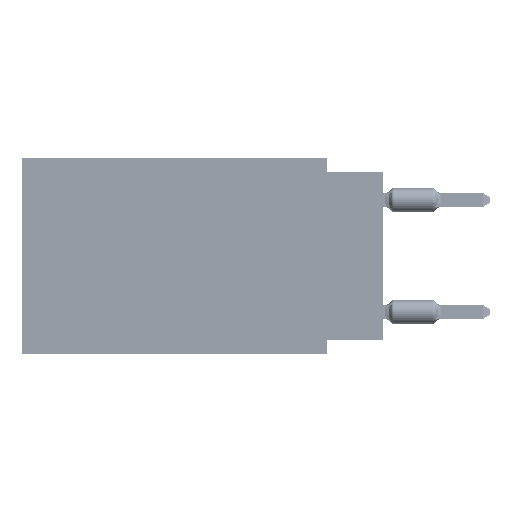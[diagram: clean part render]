
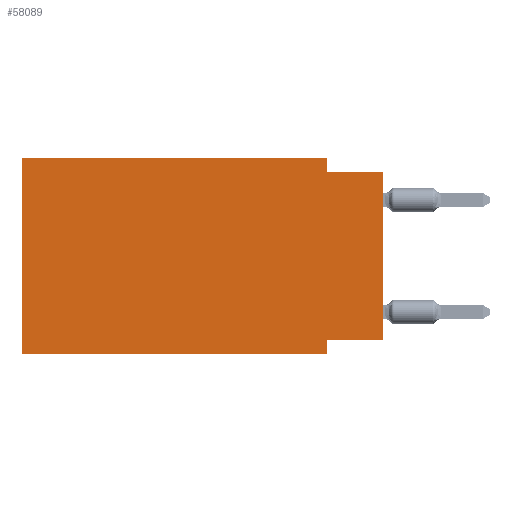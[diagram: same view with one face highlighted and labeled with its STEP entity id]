
A CAD part, left-side view. The second image highlights one B-rep face of the part: STEP entity #58089.
In plain terms, the highlighted planar face has unit normal (-1, 0, 0).
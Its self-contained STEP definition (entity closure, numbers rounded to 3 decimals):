
#378 = PLANE ( 'NONE',  #42816 ) ;
#550 = DIRECTION ( 'NONE',  ( 0., -1., 0. ) ) ;
#5020 = VERTEX_POINT ( 'NONE', #30800 ) ;
#8873 = CARTESIAN_POINT ( 'NONE',  ( 0., 0., -8.255 ) ) ;
#9636 = VECTOR ( 'NONE', #550, 1000. ) ;
#10598 = CARTESIAN_POINT ( 'NONE',  ( 0., 16.383, 0. ) ) ;
#11968 = DIRECTION ( 'NONE',  ( 0., -1., 0. ) ) ;
#13054 = VERTEX_POINT ( 'NONE', #8873 ) ;
#13843 = CARTESIAN_POINT ( 'NONE',  ( 0., 0., 0. ) ) ;
#15444 = FACE_OUTER_BOUND ( 'NONE', #65010, .T. ) ;
#16419 = CARTESIAN_POINT ( 'NONE',  ( 0., 2.54, 0. ) ) ;
#16460 = ORIENTED_EDGE ( 'NONE', *, *, #53883, .T. ) ;
#17053 = CARTESIAN_POINT ( 'NONE',  ( 0., 16.383, -8.89 ) ) ;
#17792 = ORIENTED_EDGE ( 'NONE', *, *, #63021, .T. ) ;
#18170 = CARTESIAN_POINT ( 'NONE',  ( 0., 16.383, 0. ) ) ;
#18852 = ORIENTED_EDGE ( 'NONE', *, *, #43404, .F. ) ;
#19345 = VECTOR ( 'NONE', #39985, 1000. ) ;
#19367 = VERTEX_POINT ( 'NONE', #58311 ) ;
#19750 = DIRECTION ( 'NONE',  ( 0., -1., 0. ) ) ;
#21547 = CARTESIAN_POINT ( 'NONE',  ( 0., 2.54, -8.89 ) ) ;
#22977 = EDGE_CURVE ( 'NONE', #44737, #38141, #67153, .T. ) ;
#23266 = ORIENTED_EDGE ( 'NONE', *, *, #51055, .F. ) ;
#24099 = EDGE_CURVE ( 'NONE', #13054, #19367, #51423, .T. ) ;
#24150 = VECTOR ( 'NONE', #27862, 1000. ) ;
#24558 = VERTEX_POINT ( 'NONE', #34213 ) ;
#25227 = VECTOR ( 'NONE', #11968, 1000. ) ;
#27592 = CARTESIAN_POINT ( 'NONE',  ( 0., 16.383, 0. ) ) ;
#27862 = DIRECTION ( 'NONE',  ( 0., 0., -1. ) ) ;
#28994 = VERTEX_POINT ( 'NONE', #45115 ) ;
#30800 = CARTESIAN_POINT ( 'NONE',  ( 0., 0., -0.635 ) ) ;
#33841 = LINE ( 'NONE', #65307, #9636 ) ;
#33950 = CARTESIAN_POINT ( 'NONE',  ( 0., 0., -8.255 ) ) ;
#34213 = CARTESIAN_POINT ( 'NONE',  ( 0., 2.54, 0. ) ) ;
#35665 = DIRECTION ( 'NONE',  ( 0., 0., 1. ) ) ;
#37138 = ORIENTED_EDGE ( 'NONE', *, *, #55417, .F. ) ;
#38141 = VERTEX_POINT ( 'NONE', #10598 ) ;
#39985 = DIRECTION ( 'NONE',  ( 0., 0., 1. ) ) ;
#40920 = VECTOR ( 'NONE', #69983, 1000. ) ;
#41528 = ORIENTED_EDGE ( 'NONE', *, *, #65542, .F. ) ;
#42106 = CARTESIAN_POINT ( 'NONE',  ( 0., 2.54, -8.89 ) ) ;
#42580 = VECTOR ( 'NONE', #35665, 1000. ) ;
#42816 = AXIS2_PLACEMENT_3D ( 'NONE', #27592, #43329, #65134 ) ;
#43329 = DIRECTION ( 'NONE',  ( 1., 0., 0. ) ) ;
#43404 = EDGE_CURVE ( 'NONE', #19367, #61245, #48171, .T. ) ;
#44174 = CARTESIAN_POINT ( 'NONE',  ( 0., 16.383, -8.89 ) ) ;
#44737 = VERTEX_POINT ( 'NONE', #17053 ) ;
#45115 = CARTESIAN_POINT ( 'NONE',  ( 0., 2.54, -0.635 ) ) ;
#45869 = CARTESIAN_POINT ( 'NONE',  ( 0., 0., -0.635 ) ) ;
#46690 = ORIENTED_EDGE ( 'NONE', *, *, #22977, .F. ) ;
#48171 = LINE ( 'NONE', #42106, #40920 ) ;
#49313 = LINE ( 'NONE', #16419, #24150 ) ;
#50774 = VECTOR ( 'NONE', #19750, 1000. ) ;
#51055 = EDGE_CURVE ( 'NONE', #28994, #5020, #56593, .T. ) ;
#51423 = LINE ( 'NONE', #33950, #66256 ) ;
#51750 = ORIENTED_EDGE ( 'NONE', *, *, #24099, .F. ) ;
#53883 = EDGE_CURVE ( 'NONE', #13054, #5020, #62824, .T. ) ;
#55417 = EDGE_CURVE ( 'NONE', #38141, #24558, #33841, .T. ) ;
#56593 = LINE ( 'NONE', #45869, #50774 ) ;
#58089 = ADVANCED_FACE ( 'NONE', ( #15444 ), #378, .F. ) ;
#58311 = CARTESIAN_POINT ( 'NONE',  ( 0., 2.54, -8.255 ) ) ;
#59915 = LINE ( 'NONE', #44174, #25227 ) ;
#61245 = VERTEX_POINT ( 'NONE', #21547 ) ;
#62824 = LINE ( 'NONE', #13843, #42580 ) ;
#63021 = EDGE_CURVE ( 'NONE', #44737, #61245, #59915, .T. ) ;
#65010 = EDGE_LOOP ( 'NONE', ( #16460, #23266, #41528, #37138, #46690, #17792, #18852, #51750 ) ) ;
#65134 = DIRECTION ( 'NONE',  ( 0., 0., -1. ) ) ;
#65307 = CARTESIAN_POINT ( 'NONE',  ( 0., 16.383, 0. ) ) ;
#65542 = EDGE_CURVE ( 'NONE', #24558, #28994, #49313, .T. ) ;
#66256 = VECTOR ( 'NONE', #67870, 1000. ) ;
#67153 = LINE ( 'NONE', #18170, #19345 ) ;
#67870 = DIRECTION ( 'NONE',  ( 0., 1., 0. ) ) ;
#69983 = DIRECTION ( 'NONE',  ( 0., 0., -1. ) ) ;
